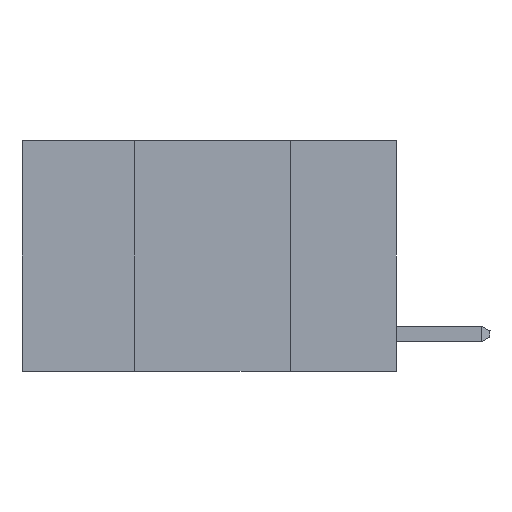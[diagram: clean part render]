
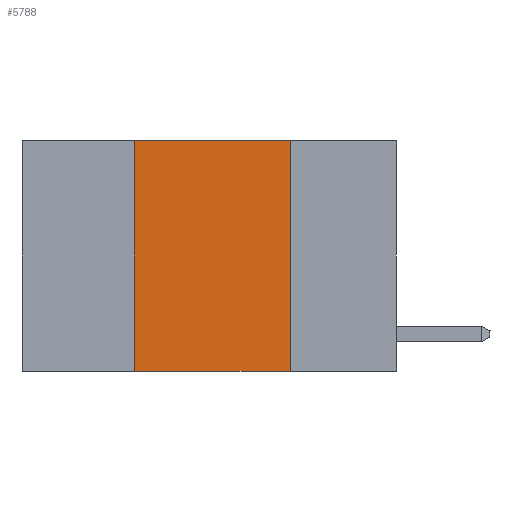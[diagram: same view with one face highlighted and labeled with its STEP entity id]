
A CAD part, left-side view. The second image highlights one B-rep face of the part: STEP entity #5788.
In plain terms, the highlighted planar face has unit normal (-1, 0, 0).
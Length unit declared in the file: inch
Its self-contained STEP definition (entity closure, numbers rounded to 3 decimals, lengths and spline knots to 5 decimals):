
#1149 = ORIENTED_EDGE ( 'NONE', *, *, #7204, .F. ) ;
#1836 = LINE ( 'NONE', #2009, #3289 ) ;
#2009 = CARTESIAN_POINT ( 'NONE',  ( 0., 0.6, 0. ) ) ;
#3222 = CARTESIAN_POINT ( 'NONE',  ( 0., 0.17, -0.37 ) ) ;
#3289 = VECTOR ( 'NONE', #11681, 39.37008 ) ;
#3311 = CARTESIAN_POINT ( 'NONE',  ( 0., 0.42, 0. ) ) ;
#4047 = CARTESIAN_POINT ( 'NONE',  ( 0., 0.42, -0.37 ) ) ;
#4735 = EDGE_CURVE ( 'NONE', #12534, #10691, #13320, .T. ) ;
#5788 = ADVANCED_FACE ( 'NONE', ( #13205 ), #7049, .F. ) ;
#6000 = DIRECTION ( 'NONE',  ( 0., 0., 1. ) ) ;
#6111 = CARTESIAN_POINT ( 'NONE',  ( 0., 0.6, -0.37 ) ) ;
#6358 = EDGE_CURVE ( 'NONE', #15760, #11018, #1836, .T. ) ;
#7049 = PLANE ( 'NONE',  #9943 ) ;
#7204 = EDGE_CURVE ( 'NONE', #11018, #10691, #9534, .T. ) ;
#7342 = EDGE_CURVE ( 'NONE', #12534, #15760, #12125, .T. ) ;
#8001 = VECTOR ( 'NONE', #11973, 39.37008 ) ;
#8011 = VECTOR ( 'NONE', #6000, 39.37008 ) ;
#9534 = LINE ( 'NONE', #10990, #8001 ) ;
#9538 = CARTESIAN_POINT ( 'NONE',  ( 0., 0.6, 0. ) ) ;
#9836 = CARTESIAN_POINT ( 'NONE',  ( 0., 0.17, 0. ) ) ;
#9943 = AXIS2_PLACEMENT_3D ( 'NONE', #9538, #15767, #14526 ) ;
#10691 = VERTEX_POINT ( 'NONE', #3222 ) ;
#10990 = CARTESIAN_POINT ( 'NONE',  ( 0., 0.17, 0. ) ) ;
#11018 = VERTEX_POINT ( 'NONE', #9836 ) ;
#11681 = DIRECTION ( 'NONE',  ( 0., -1., 0. ) ) ;
#11816 = VECTOR ( 'NONE', #14800, 39.37008 ) ;
#11973 = DIRECTION ( 'NONE',  ( 0., 0., -1. ) ) ;
#12125 = LINE ( 'NONE', #14760, #8011 ) ;
#12534 = VERTEX_POINT ( 'NONE', #4047 ) ;
#12541 = EDGE_LOOP ( 'NONE', ( #1149, #15806, #15620, #14379 ) ) ;
#13205 = FACE_OUTER_BOUND ( 'NONE', #12541, .T. ) ;
#13320 = LINE ( 'NONE', #6111, #11816 ) ;
#14379 = ORIENTED_EDGE ( 'NONE', *, *, #4735, .T. ) ;
#14526 = DIRECTION ( 'NONE',  ( 0., 0., -1. ) ) ;
#14760 = CARTESIAN_POINT ( 'NONE',  ( 0., 0.42, 0. ) ) ;
#14800 = DIRECTION ( 'NONE',  ( 0., -1., 0. ) ) ;
#15620 = ORIENTED_EDGE ( 'NONE', *, *, #7342, .F. ) ;
#15760 = VERTEX_POINT ( 'NONE', #3311 ) ;
#15767 = DIRECTION ( 'NONE',  ( 1., 0., 0. ) ) ;
#15806 = ORIENTED_EDGE ( 'NONE', *, *, #6358, .F. ) ;
